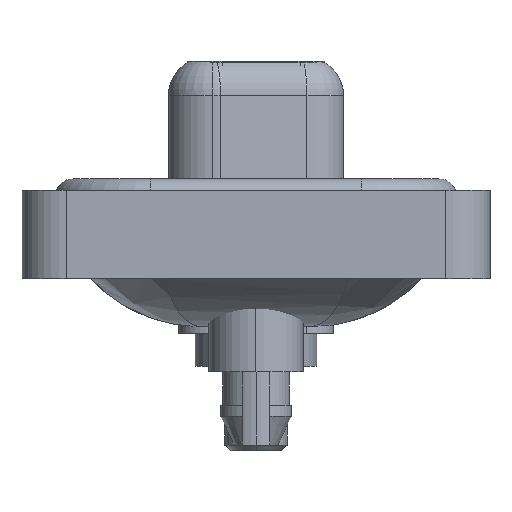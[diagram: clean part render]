
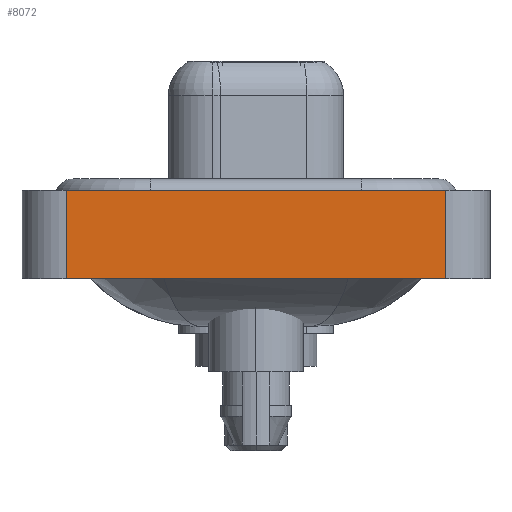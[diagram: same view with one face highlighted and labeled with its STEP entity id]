
A CAD part, left-side view. The second image highlights one B-rep face of the part: STEP entity #8072.
In plain terms, the highlighted planar face has unit normal (-1, 0, 0).
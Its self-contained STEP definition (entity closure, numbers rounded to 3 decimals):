
#79 = DIRECTION ( 'NONE',  ( -1., 0., 0. ) ) ;
#625 = ORIENTED_EDGE ( 'NONE', *, *, #10057, .T. ) ;
#2768 = PLANE ( 'NONE',  #13034 ) ;
#3148 = ORIENTED_EDGE ( 'NONE', *, *, #11331, .F. ) ;
#3736 = DIRECTION ( 'NONE',  ( 0., 0., 1. ) ) ;
#3819 = VERTEX_POINT ( 'NONE', #16061 ) ;
#5107 = CARTESIAN_POINT ( 'NONE',  ( -7.25, -8.55, -3.6 ) ) ;
#5297 = EDGE_CURVE ( 'NONE', #3819, #9342, #12506, .T. ) ;
#5373 = VERTEX_POINT ( 'NONE', #8694 ) ;
#6496 = CARTESIAN_POINT ( 'NONE',  ( -7.25, 8.55, -3.6 ) ) ;
#6570 = CARTESIAN_POINT ( 'NONE',  ( -7.25, -8.55, 0.4 ) ) ;
#6579 = VECTOR ( 'NONE', #9724, 1000. ) ;
#6819 = VECTOR ( 'NONE', #3736, 1000. ) ;
#6922 = EDGE_LOOP ( 'NONE', ( #15062, #3148, #16524, #625 ) ) ;
#7948 = LINE ( 'NONE', #5107, #16594 ) ;
#8072 = ADVANCED_FACE ( 'NONE', ( #15470 ), #2768, .T. ) ;
#8221 = VERTEX_POINT ( 'NONE', #9499 ) ;
#8694 = CARTESIAN_POINT ( 'NONE',  ( -7.25, 8.55, 0.4 ) ) ;
#9285 = DIRECTION ( 'NONE',  ( 0., -1., 0. ) ) ;
#9342 = VERTEX_POINT ( 'NONE', #6570 ) ;
#9499 = CARTESIAN_POINT ( 'NONE',  ( -7.25, 8.55, -3.6 ) ) ;
#9724 = DIRECTION ( 'NONE',  ( 0., 0., 1. ) ) ;
#10057 = EDGE_CURVE ( 'NONE', #8221, #3819, #7948, .T. ) ;
#10433 = VECTOR ( 'NONE', #11715, 1000. ) ;
#10686 = LINE ( 'NONE', #6496, #6819 ) ;
#11331 = EDGE_CURVE ( 'NONE', #5373, #9342, #11522, .T. ) ;
#11522 = LINE ( 'NONE', #14497, #10433 ) ;
#11715 = DIRECTION ( 'NONE',  ( 0., -1., 0. ) ) ;
#12506 = LINE ( 'NONE', #18198, #6579 ) ;
#12674 = DIRECTION ( 'NONE',  ( 0., 0., 1. ) ) ;
#13034 = AXIS2_PLACEMENT_3D ( 'NONE', #14090, #79, #12674 ) ;
#14090 = CARTESIAN_POINT ( 'NONE',  ( -7.25, -8.55, -3.6 ) ) ;
#14497 = CARTESIAN_POINT ( 'NONE',  ( -7.25, -8.55, 0.4 ) ) ;
#15062 = ORIENTED_EDGE ( 'NONE', *, *, #5297, .T. ) ;
#15470 = FACE_OUTER_BOUND ( 'NONE', #6922, .T. ) ;
#16061 = CARTESIAN_POINT ( 'NONE',  ( -7.25, -8.55, -3.6 ) ) ;
#16524 = ORIENTED_EDGE ( 'NONE', *, *, #16877, .F. ) ;
#16594 = VECTOR ( 'NONE', #9285, 1000. ) ;
#16877 = EDGE_CURVE ( 'NONE', #8221, #5373, #10686, .T. ) ;
#18198 = CARTESIAN_POINT ( 'NONE',  ( -7.25, -8.55, -3.6 ) ) ;
